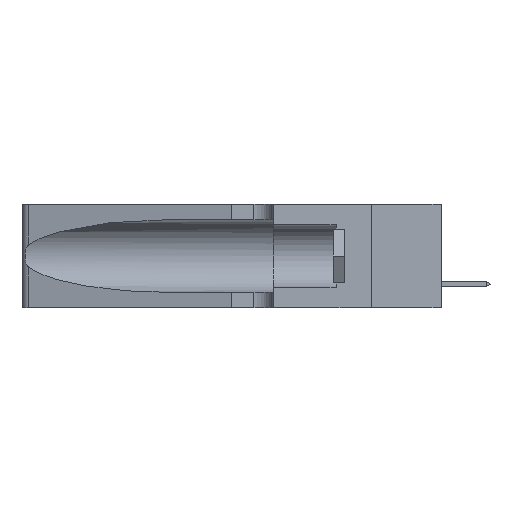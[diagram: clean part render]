
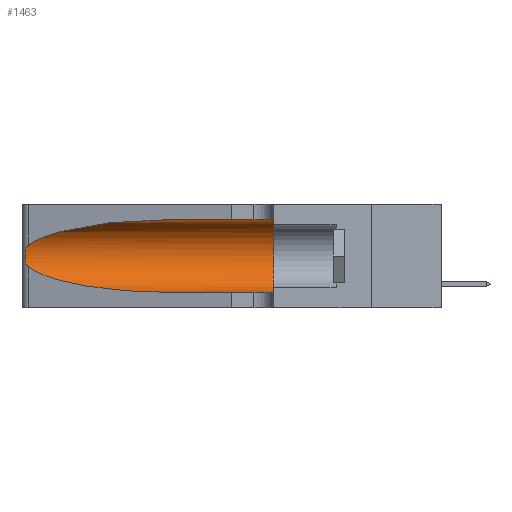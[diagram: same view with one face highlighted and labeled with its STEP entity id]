
A CAD part, left-side view. The second image highlights one B-rep face of the part: STEP entity #1463.
In plain terms, the highlighted cylindrical face has radius 3.308 mm (diameter 6.617 mm), a partial arc.
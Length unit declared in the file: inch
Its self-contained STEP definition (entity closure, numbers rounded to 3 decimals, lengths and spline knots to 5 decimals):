
#207 = CARTESIAN_POINT ( 'NONE',  ( 0.25487, 1.22718, 0.14631 ) ) ;
#1463 = ADVANCED_FACE ( 'NONE', ( #12111 ), #27016, .F. ) ;
#1566 = ORIENTED_EDGE ( 'NONE', *, *, #14772, .T. ) ;
#1734 = ORIENTED_EDGE ( 'NONE', *, *, #16451, .T. ) ;
#3230 = CARTESIAN_POINT ( 'NONE',  ( 0.2373, 1.15595, 0.08982 ) ) ;
#3298 = LINE ( 'NONE', #4232, #12107 ) ;
#4232 = CARTESIAN_POINT ( 'NONE',  ( 0.1305, 1.61858, 0.31525 ) ) ;
#4393 = VERTEX_POINT ( 'NONE', #5606 ) ;
#4519 = CARTESIAN_POINT ( 'NONE',  ( 0.26018, 1.23835, 0.19895 ) ) ;
#4607 = CIRCLE ( 'NONE', #19093, 0.13025 ) ;
#5028 = CARTESIAN_POINT ( 'NONE',  ( 0.1305, 1.61858, 0.05475 ) ) ;
#5380 = AXIS2_PLACEMENT_3D ( 'NONE', #19167, #30148, #27922 ) ;
#5606 = CARTESIAN_POINT ( 'NONE',  ( 0.1305, 0.72297, 0.05475 ) ) ;
#6552 = CARTESIAN_POINT ( 'NONE',  ( 0.25487, 1.22718, 0.22369 ) ) ;
#6661 = VERTEX_POINT ( 'NONE', #29644 ) ;
#6664 = CARTESIAN_POINT ( 'NONE',  ( 0.25854, 1.2359, 0.20912 ) ) ;
#7235 = CARTESIAN_POINT ( 'NONE',  ( 0.25555, 1.22993, 0.14849 ) ) ;
#7707 = CARTESIAN_POINT ( 'NONE',  ( 0.18966, 0.96281, 0.31525 ) ) ;
#7751 = CARTESIAN_POINT ( 'NONE',  ( 0.1305, 0.72297, 0.05475 ) ) ;
#7818 = CARTESIAN_POINT ( 'NONE',  ( 0.25487, 1.22718, 0.22369 ) ) ;
#9039 = CARTESIAN_POINT ( 'NONE',  ( 0.26075, 1.23896, 0.19203 ) ) ;
#10156 = CARTESIAN_POINT ( 'NONE',  ( 0.25487, 1.22718, 0.22369 ) ) ;
#10815 = EDGE_LOOP ( 'NONE', ( #24454, #23505, #1566, #1734, #25595, #21837 ) ) ;
#11075 = CARTESIAN_POINT ( 'NONE',  ( 0.18966, 0.96281, 0.05475 ) ) ;
#11416 = CARTESIAN_POINT ( 'NONE',  ( 0.26075, 1.23896, 0.178 ) ) ;
#12107 = VECTOR ( 'NONE', #15500, 39.37008 ) ;
#12111 = FACE_OUTER_BOUND ( 'NONE', #10815, .T. ) ;
#12226 = VERTEX_POINT ( 'NONE', #19633 ) ;
#14217 = CARTESIAN_POINT ( 'NONE',  ( 0.25639, 1.23186, 0.15144 ) ) ;
#14513 = CARTESIAN_POINT ( 'NONE',  ( 0.25789, 1.23486, 0.15765 ) ) ;
#14660 = CARTESIAN_POINT ( 'NONE',  ( 0.1305, 0.72297, 0.31525 ) ) ;
#14772 = EDGE_CURVE ( 'NONE', #21139, #4393, #23753, .T. ) ;
#15500 = DIRECTION ( 'NONE',  ( 0., -1., 0. ) ) ;
#16364 = CARTESIAN_POINT ( 'NONE',  ( 0.25787, 1.23484, 0.2124 ) ) ;
#16451 = EDGE_CURVE ( 'NONE', #4393, #12226, #21746, .T. ) ;
#16581 = EDGE_CURVE ( 'NONE', #29407, #12226, #4607, .T. ) ;
#17008 = VECTOR ( 'NONE', #21058, 39.37008 ) ;
#17407 = CARTESIAN_POINT ( 'NONE',  ( 0.25487, 1.22718, 0.14631 ) ) ;
#18353 =( BOUNDED_CURVE ( )  B_SPLINE_CURVE ( 3, ( #14660, #7707, #24028, #7818 ),
 .UNSPECIFIED., .F., .F. ) 
 B_SPLINE_CURVE_WITH_KNOTS ( ( 4, 4 ),
 ( 1.5708, 2.84003 ),
 .UNSPECIFIED. ) 
 CURVE ( )  GEOMETRIC_REPRESENTATION_ITEM ( )  RATIONAL_B_SPLINE_CURVE ( ( 1., 0.87, 0.87, 1. ) ) 
 REPRESENTATION_ITEM ( '' )  );
#19093 = AXIS2_PLACEMENT_3D ( 'NONE', #22503, #27449, #27044 ) ;
#19167 = CARTESIAN_POINT ( 'NONE',  ( 0.1305, 1.61858, 0.185 ) ) ;
#19633 = CARTESIAN_POINT ( 'NONE',  ( 0.1305, 0.35, 0.05475 ) ) ;
#20495 = EDGE_CURVE ( 'NONE', #6661, #29407, #3298, .T. ) ;
#21025 = CARTESIAN_POINT ( 'NONE',  ( 0.26017, 1.23833, 0.17102 ) ) ;
#21058 = DIRECTION ( 'NONE',  ( 0., -1., 0. ) ) ;
#21139 = VERTEX_POINT ( 'NONE', #23046 ) ;
#21215 = CARTESIAN_POINT ( 'NONE',  ( 0.25856, 1.23593, 0.16098 ) ) ;
#21417 = CARTESIAN_POINT ( 'NONE',  ( 0.25555, 1.22994, 0.2215 ) ) ;
#21746 = LINE ( 'NONE', #5028, #17008 ) ;
#21837 = ORIENTED_EDGE ( 'NONE', *, *, #20495, .F. ) ;
#22503 = CARTESIAN_POINT ( 'NONE',  ( 0.1305, 0.35, 0.185 ) ) ;
#23046 = CARTESIAN_POINT ( 'NONE',  ( 0.25487, 1.22718, 0.14631 ) ) ;
#23505 = ORIENTED_EDGE ( 'NONE', *, *, #25663, .T. ) ;
#23721 = B_SPLINE_CURVE_WITH_KNOTS ( 'NONE', 3,
 ( #10156, #21417, #29777, #16364, #6664, #4519, #9039, #11416, #21025, #21215, #14513, #14217, #7235, #207 ),
 .UNSPECIFIED., .F., .F.,
 ( 4, 2, 2, 2, 2, 2, 4 ),
 ( 0., 0.00027, 0.00053, 0.00107, 0.0016, 0.00187, 0.00214 ),
 .UNSPECIFIED. ) ;
#23753 =( BOUNDED_CURVE ( )  B_SPLINE_CURVE ( 3, ( #17407, #3230, #11075, #7751 ),
 .UNSPECIFIED., .F., .F. ) 
 B_SPLINE_CURVE_WITH_KNOTS ( ( 4, 4 ),
 ( 3.44316, 4.71239 ),
 .UNSPECIFIED. ) 
 CURVE ( )  GEOMETRIC_REPRESENTATION_ITEM ( )  RATIONAL_B_SPLINE_CURVE ( ( 1., 0.87, 0.87, 1. ) ) 
 REPRESENTATION_ITEM ( '' )  );
#24028 = CARTESIAN_POINT ( 'NONE',  ( 0.2373, 1.15595, 0.28018 ) ) ;
#24454 = ORIENTED_EDGE ( 'NONE', *, *, #28104, .T. ) ;
#25025 = VERTEX_POINT ( 'NONE', #6552 ) ;
#25428 = CARTESIAN_POINT ( 'NONE',  ( 0.1305, 0.35, 0.31525 ) ) ;
#25595 = ORIENTED_EDGE ( 'NONE', *, *, #16581, .F. ) ;
#25663 = EDGE_CURVE ( 'NONE', #25025, #21139, #23721, .T. ) ;
#27016 = CYLINDRICAL_SURFACE ( 'NONE', #5380, 0.13025 ) ;
#27044 = DIRECTION ( 'NONE',  ( 0., 0., 1. ) ) ;
#27449 = DIRECTION ( 'NONE',  ( 0., 1., 0. ) ) ;
#27922 = DIRECTION ( 'NONE',  ( 0., 0., -1. ) ) ;
#28104 = EDGE_CURVE ( 'NONE', #6661, #25025, #18353, .T. ) ;
#29407 = VERTEX_POINT ( 'NONE', #25428 ) ;
#29644 = CARTESIAN_POINT ( 'NONE',  ( 0.1305, 0.72297, 0.31525 ) ) ;
#29777 = CARTESIAN_POINT ( 'NONE',  ( 0.25639, 1.23184, 0.21858 ) ) ;
#30148 = DIRECTION ( 'NONE',  ( 0., -1., 0. ) ) ;
